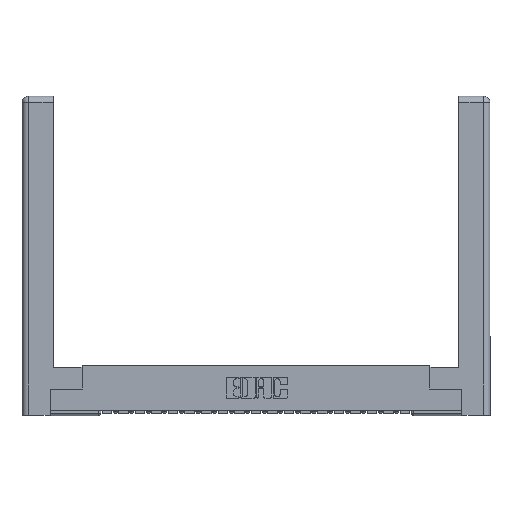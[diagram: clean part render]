
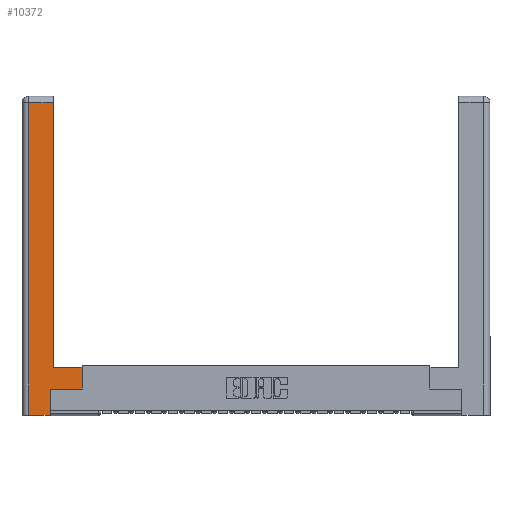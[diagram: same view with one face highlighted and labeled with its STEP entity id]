
A CAD part, top view. The second image highlights one B-rep face of the part: STEP entity #10372.
In plain terms, the highlighted planar face has unit normal (0, 0, 1).
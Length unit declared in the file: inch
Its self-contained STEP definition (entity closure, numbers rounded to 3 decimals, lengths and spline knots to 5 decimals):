
#4 = EDGE_CURVE ( 'NONE', #1798, #5031, #10451, .T. ) ;
#254 = DIRECTION ( 'NONE',  ( 0., 0., -1. ) ) ;
#422 = CARTESIAN_POINT ( 'NONE',  ( 0.565, 0.245, 0. ) ) ;
#783 = FACE_OUTER_BOUND ( 'NONE', #5996, .T. ) ;
#1194 = LINE ( 'NONE', #9358, #9402 ) ;
#1798 = VERTEX_POINT ( 'NONE', #13163 ) ;
#1889 = ORIENTED_EDGE ( 'NONE', *, *, #4, .T. ) ;
#2009 = VECTOR ( 'NONE', #13078, 39.37008 ) ;
#2160 = CARTESIAN_POINT ( 'NONE',  ( 0.265, 0., 0. ) ) ;
#3083 = VECTOR ( 'NONE', #7500, 39.37008 ) ;
#3278 = ORIENTED_EDGE ( 'NONE', *, *, #20338, .T. ) ;
#3363 = ORIENTED_EDGE ( 'NONE', *, *, #4609, .T. ) ;
#3640 = LINE ( 'NONE', #2160, #3083 ) ;
#4373 = DIRECTION ( 'NONE',  ( -1., 0., 0. ) ) ;
#4397 = CARTESIAN_POINT ( 'NONE',  ( 0.565, 0.45, 0. ) ) ;
#4609 = EDGE_CURVE ( 'NONE', #16011, #16627, #3640, .T. ) ;
#5031 = VERTEX_POINT ( 'NONE', #9971 ) ;
#5202 = VERTEX_POINT ( 'NONE', #13298 ) ;
#5242 = LINE ( 'NONE', #12356, #14310 ) ;
#5594 = VERTEX_POINT ( 'NONE', #9502 ) ;
#5996 = EDGE_LOOP ( 'NONE', ( #14866, #1889, #15904, #3363, #3278, #8478, #7598, #6663 ) ) ;
#6663 = ORIENTED_EDGE ( 'NONE', *, *, #15848, .T. ) ;
#7131 = EDGE_CURVE ( 'NONE', #5031, #16011, #17174, .T. ) ;
#7334 = DIRECTION ( 'NONE',  ( 0., 1., 0. ) ) ;
#7366 = VERTEX_POINT ( 'NONE', #15303 ) ;
#7500 = DIRECTION ( 'NONE',  ( 1., 0., 0. ) ) ;
#7598 = ORIENTED_EDGE ( 'NONE', *, *, #13641, .T. ) ;
#7607 = PLANE ( 'NONE',  #14802 ) ;
#7717 = EDGE_CURVE ( 'NONE', #5594, #1798, #1194, .T. ) ;
#8478 = ORIENTED_EDGE ( 'NONE', *, *, #10442, .T. ) ;
#9358 = CARTESIAN_POINT ( 'NONE',  ( 0.295, 3., 0. ) ) ;
#9402 = VECTOR ( 'NONE', #7334, 39.37008 ) ;
#9502 = CARTESIAN_POINT ( 'NONE',  ( 0.295, 0.45, 0. ) ) ;
#9744 = CARTESIAN_POINT ( 'NONE',  ( 0.0615, 2.94, 0. ) ) ;
#9822 = VERTEX_POINT ( 'NONE', #422 ) ;
#9971 = CARTESIAN_POINT ( 'NONE',  ( 0.0615, 2.94, 0. ) ) ;
#10372 = ADVANCED_FACE ( 'NONE', ( #783 ), #7607, .F. ) ;
#10442 = EDGE_CURVE ( 'NONE', #7366, #9822, #13413, .T. ) ;
#10451 = LINE ( 'NONE', #9744, #12374 ) ;
#10980 = DIRECTION ( 'NONE',  ( -1., 0., 0. ) ) ;
#11129 = VECTOR ( 'NONE', #10980, 39.37008 ) ;
#11259 = CARTESIAN_POINT ( 'NONE',  ( 0.265, 0., 0. ) ) ;
#11269 = DIRECTION ( 'NONE',  ( 1., 0., 0. ) ) ;
#11378 = CARTESIAN_POINT ( 'NONE',  ( 0.0615, 0., 0. ) ) ;
#11383 = DIRECTION ( 'NONE',  ( 0., 1., 0. ) ) ;
#11968 = LINE ( 'NONE', #21485, #11129 ) ;
#12356 = CARTESIAN_POINT ( 'NONE',  ( 0.265, 0.245, 0. ) ) ;
#12374 = VECTOR ( 'NONE', #4373, 39.37008 ) ;
#12645 = DIRECTION ( 'NONE',  ( 0., 1., 0. ) ) ;
#13078 = DIRECTION ( 'NONE',  ( 0., -1., 0. ) ) ;
#13163 = CARTESIAN_POINT ( 'NONE',  ( 0.295, 2.94, 0. ) ) ;
#13298 = CARTESIAN_POINT ( 'NONE',  ( 0.565, 0.45, 0. ) ) ;
#13413 = LINE ( 'NONE', #14520, #18634 ) ;
#13641 = EDGE_CURVE ( 'NONE', #9822, #5202, #19943, .T. ) ;
#14310 = VECTOR ( 'NONE', #12645, 39.37008 ) ;
#14369 = CARTESIAN_POINT ( 'NONE',  ( 0., 0., 0. ) ) ;
#14520 = CARTESIAN_POINT ( 'NONE',  ( 0.565, 0.245, 0. ) ) ;
#14802 = AXIS2_PLACEMENT_3D ( 'NONE', #14369, #254, #21407 ) ;
#14866 = ORIENTED_EDGE ( 'NONE', *, *, #7717, .T. ) ;
#15303 = CARTESIAN_POINT ( 'NONE',  ( 0.265, 0.245, 0. ) ) ;
#15848 = EDGE_CURVE ( 'NONE', #5202, #5594, #11968, .T. ) ;
#15904 = ORIENTED_EDGE ( 'NONE', *, *, #7131, .T. ) ;
#16011 = VERTEX_POINT ( 'NONE', #18274 ) ;
#16627 = VERTEX_POINT ( 'NONE', #11259 ) ;
#17174 = LINE ( 'NONE', #11378, #2009 ) ;
#17189 = VECTOR ( 'NONE', #11383, 39.37008 ) ;
#18274 = CARTESIAN_POINT ( 'NONE',  ( 0.0615, 0., 0. ) ) ;
#18634 = VECTOR ( 'NONE', #11269, 39.37008 ) ;
#19943 = LINE ( 'NONE', #4397, #17189 ) ;
#20338 = EDGE_CURVE ( 'NONE', #16627, #7366, #5242, .T. ) ;
#21407 = DIRECTION ( 'NONE',  ( -1., 0., 0. ) ) ;
#21485 = CARTESIAN_POINT ( 'NONE',  ( 0.295, 0.45, 0. ) ) ;
